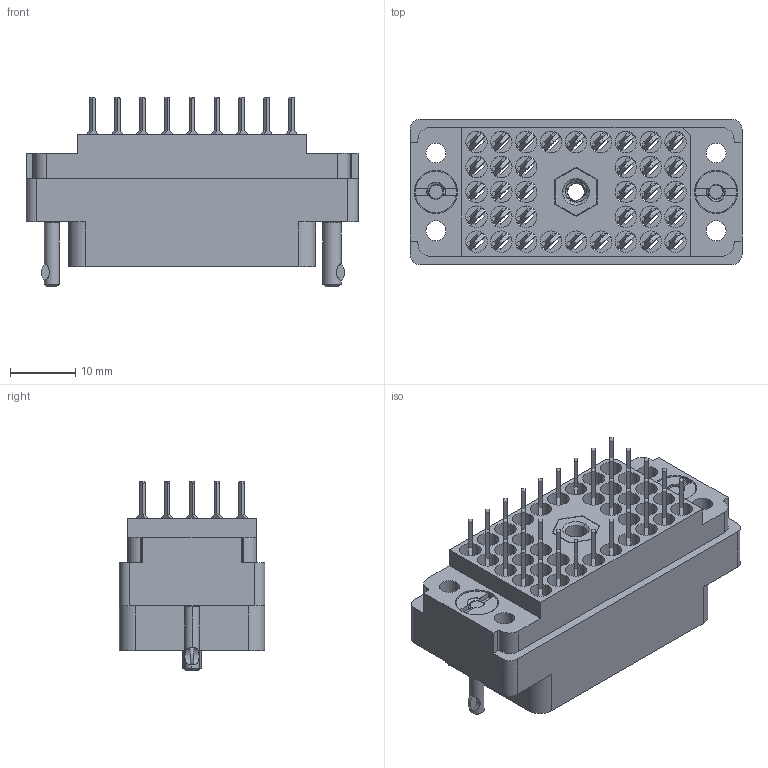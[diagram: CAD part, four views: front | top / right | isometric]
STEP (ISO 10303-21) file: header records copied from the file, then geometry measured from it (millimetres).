
FILE_DESCRIPTION (( 'STEP AP203' ), '1' );
FILE_NAME ('519-036-520-302.STEP', '2020-03-11T16:12:18', ( '' ), ( '' ), 'SwSTEP 2.0', 'SolidWorks 2016', '' );
FILE_SCHEMA (( 'CONFIG_CONTROL_DESIGN' ));
Length unit declared in the file: inch
Products named in the file (7): 516-252-021-102_038; 516-222-038-102_038; 516-252-035-100_516-252-035-100; 516-292-001_520 Contact; 519 Plug Insulator_036; 516-222-038-102_039; 519-036-520-302
Assembly tree (42 placements, depth 2):
  519-036-520-302
    519 Plug Insulator_036
    516-292-001_520 Contact  x36
    516-252-035-100_516-252-035-100
    516-252-021-102_038  x2
    516-222-038-102_038
    516-222-038-102_039
Bounding box: 50.8 x 22.25 x 29.01 mm (x, y, z)
Volume: 10760.6 mm3; surface area: 18480.7 mm2
Topology: 42 solids, 42 shells, 3684 faces, 10599 edges, 7022 vertices
Faces by surface type: plane 2182, cylinder 1194, bspline 258, cone 46, torus 4
Entity records: 45672 total; most frequent: CARTESIAN_POINT 14071, ORIENTED_EDGE 6458, DIRECTION 6055, EDGE_CURVE 3229, VECTOR 2163, LINE 2163, VERTEX_POINT 2132, AXIS2_PLACEMENT_3D 1946
